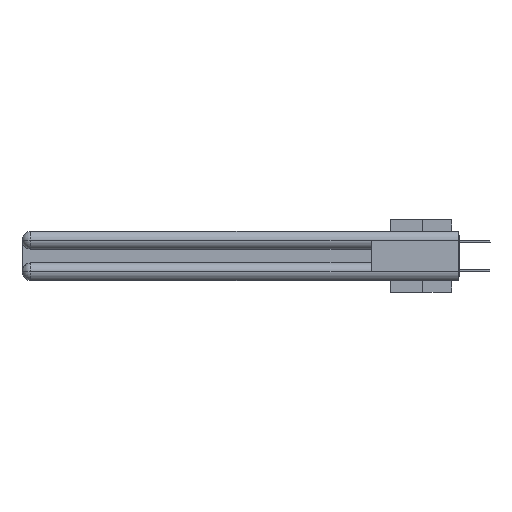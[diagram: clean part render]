
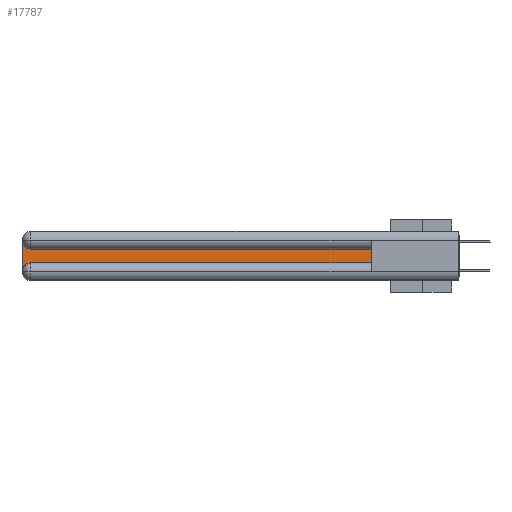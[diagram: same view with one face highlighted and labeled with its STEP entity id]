
A CAD part, left-side view. The second image highlights one B-rep face of the part: STEP entity #17787.
In plain terms, the highlighted planar face has unit normal (-1, 0, 0).
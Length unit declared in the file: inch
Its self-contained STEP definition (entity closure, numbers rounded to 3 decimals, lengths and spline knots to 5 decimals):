
#41 = AXIS2_PLACEMENT_3D ( 'NONE', #14605, #28975, #23178 ) ;
#526 = CARTESIAN_POINT ( 'NONE',  ( 0.075, 3., -0.2175 ) ) ;
#696 = LINE ( 'NONE', #28931, #18029 ) ;
#1978 = VERTEX_POINT ( 'NONE', #18540 ) ;
#2602 = CIRCLE ( 'NONE', #22925, 0.06 ) ;
#3315 = VECTOR ( 'NONE', #16560, 39.37008 ) ;
#3907 = CARTESIAN_POINT ( 'NONE',  ( 0.075, 3., -0.1225 ) ) ;
#4589 = VERTEX_POINT ( 'NONE', #18286 ) ;
#5044 = DIRECTION ( 'NONE',  ( 1., 0., 0. ) ) ;
#5110 = CARTESIAN_POINT ( 'NONE',  ( 0.075, 0.6, -0.2175 ) ) ;
#7456 = PLANE ( 'NONE',  #19414 ) ;
#9499 = VERTEX_POINT ( 'NONE', #33836 ) ;
#11244 = DIRECTION ( 'NONE',  ( 0., 0., -1. ) ) ;
#11409 = VECTOR ( 'NONE', #20764, 39.37008 ) ;
#11963 = DIRECTION ( 'NONE',  ( 0., 0., -1. ) ) ;
#12672 = VECTOR ( 'NONE', #11963, 39.37008 ) ;
#13761 = EDGE_CURVE ( 'NONE', #9499, #36349, #14775, .T. ) ;
#13820 = CIRCLE ( 'NONE', #41, 0.06 ) ;
#14605 = CARTESIAN_POINT ( 'NONE',  ( 0.075, 2.94, -0.2775 ) ) ;
#14775 = LINE ( 'NONE', #526, #12672 ) ;
#15250 = CARTESIAN_POINT ( 'NONE',  ( 0.075, 2.94, -0.2175 ) ) ;
#15360 = FACE_OUTER_BOUND ( 'NONE', #28676, .T. ) ;
#16560 = DIRECTION ( 'NONE',  ( 0., -1., 0. ) ) ;
#16602 = ORIENTED_EDGE ( 'NONE', *, *, #30841, .T. ) ;
#17008 = DIRECTION ( 'NONE',  ( 0., 0., 1. ) ) ;
#17582 = ORIENTED_EDGE ( 'NONE', *, *, #36333, .T. ) ;
#17787 = ADVANCED_FACE ( 'NONE', ( #15360 ), #7456, .F. ) ;
#18029 = VECTOR ( 'NONE', #17008, 39.37008 ) ;
#18286 = CARTESIAN_POINT ( 'NONE',  ( 0.075, 0.6, -0.1225 ) ) ;
#18540 = CARTESIAN_POINT ( 'NONE',  ( 0.075, 2.94, -0.1225 ) ) ;
#19377 = LINE ( 'NONE', #5110, #3315 ) ;
#19414 = AXIS2_PLACEMENT_3D ( 'NONE', #3907, #24469, #35473 ) ;
#20399 = LINE ( 'NONE', #29511, #11409 ) ;
#20764 = DIRECTION ( 'NONE',  ( 0., 1., 0. ) ) ;
#20983 = CARTESIAN_POINT ( 'NONE',  ( 0.075, 0.6, -0.2175 ) ) ;
#21969 = VERTEX_POINT ( 'NONE', #20983 ) ;
#22747 = VERTEX_POINT ( 'NONE', #15250 ) ;
#22925 = AXIS2_PLACEMENT_3D ( 'NONE', #25076, #5044, #11244 ) ;
#23178 = DIRECTION ( 'NONE',  ( 0., 0., -1. ) ) ;
#24469 = DIRECTION ( 'NONE',  ( 1., 0., 0. ) ) ;
#25076 = CARTESIAN_POINT ( 'NONE',  ( 0.075, 2.94, -0.0625 ) ) ;
#26322 = ORIENTED_EDGE ( 'NONE', *, *, #32814, .T. ) ;
#26357 = EDGE_CURVE ( 'NONE', #36349, #22747, #13820, .T. ) ;
#26917 = EDGE_CURVE ( 'NONE', #21969, #4589, #696, .T. ) ;
#28676 = EDGE_LOOP ( 'NONE', ( #17582, #16602, #34996, #34719, #26322, #32522 ) ) ;
#28931 = CARTESIAN_POINT ( 'NONE',  ( 0.075, 0.6, -0.2175 ) ) ;
#28975 = DIRECTION ( 'NONE',  ( 1., 0., 0. ) ) ;
#29511 = CARTESIAN_POINT ( 'NONE',  ( 0.075, 0.6, -0.1225 ) ) ;
#30841 = EDGE_CURVE ( 'NONE', #1978, #9499, #2602, .T. ) ;
#32522 = ORIENTED_EDGE ( 'NONE', *, *, #26917, .T. ) ;
#32814 = EDGE_CURVE ( 'NONE', #22747, #21969, #19377, .T. ) ;
#33836 = CARTESIAN_POINT ( 'NONE',  ( 0.075, 3., -0.0625 ) ) ;
#34719 = ORIENTED_EDGE ( 'NONE', *, *, #26357, .T. ) ;
#34909 = CARTESIAN_POINT ( 'NONE',  ( 0.075, 3., -0.2775 ) ) ;
#34996 = ORIENTED_EDGE ( 'NONE', *, *, #13761, .T. ) ;
#35473 = DIRECTION ( 'NONE',  ( 0., 0., -1. ) ) ;
#36333 = EDGE_CURVE ( 'NONE', #4589, #1978, #20399, .T. ) ;
#36349 = VERTEX_POINT ( 'NONE', #34909 ) ;
